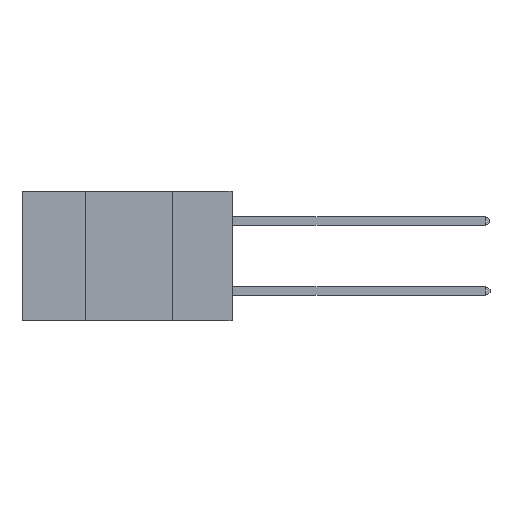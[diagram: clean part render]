
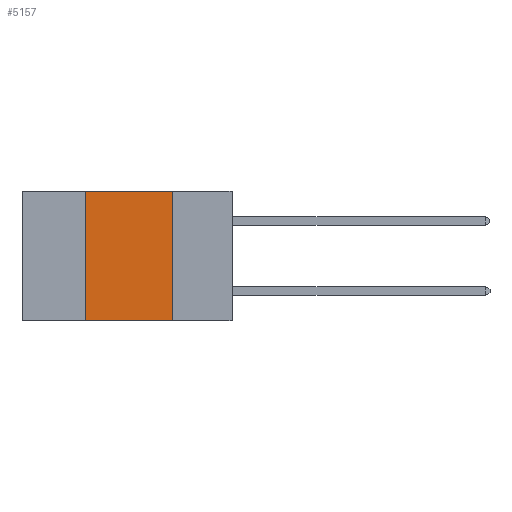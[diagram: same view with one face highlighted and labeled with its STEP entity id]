
A CAD part, left-side view. The second image highlights one B-rep face of the part: STEP entity #5157.
In plain terms, the highlighted planar face has unit normal (-1, 0, 0).
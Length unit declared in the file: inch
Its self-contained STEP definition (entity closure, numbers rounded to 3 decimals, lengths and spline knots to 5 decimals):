
#440 = CARTESIAN_POINT ( 'NONE',  ( 0., 0.17, 0. ) ) ;
#542 = LINE ( 'NONE', #7046, #11362 ) ;
#865 = VECTOR ( 'NONE', #4692, 39.37008 ) ;
#1323 = VECTOR ( 'NONE', #11215, 39.37008 ) ;
#1494 = CARTESIAN_POINT ( 'NONE',  ( 0., 0.42, 0. ) ) ;
#1680 = ORIENTED_EDGE ( 'NONE', *, *, #3179, .T. ) ;
#2598 = VERTEX_POINT ( 'NONE', #9716 ) ;
#2772 = LINE ( 'NONE', #6446, #13389 ) ;
#2850 = CARTESIAN_POINT ( 'NONE',  ( 0., 0.6, 0. ) ) ;
#3138 = EDGE_CURVE ( 'NONE', #6666, #8496, #542, .T. ) ;
#3179 = EDGE_CURVE ( 'NONE', #6666, #6652, #2772, .T. ) ;
#3407 = DIRECTION ( 'NONE',  ( 0., -1., 0. ) ) ;
#3831 = LINE ( 'NONE', #5006, #1323 ) ;
#3889 = DIRECTION ( 'NONE',  ( 0., 0., -1. ) ) ;
#3923 = EDGE_CURVE ( 'NONE', #2598, #6652, #4051, .T. ) ;
#4051 = LINE ( 'NONE', #440, #865 ) ;
#4070 = EDGE_CURVE ( 'NONE', #8496, #2598, #3831, .T. ) ;
#4692 = DIRECTION ( 'NONE',  ( 0., 0., -1. ) ) ;
#5006 = CARTESIAN_POINT ( 'NONE',  ( 0., 0.6, 0. ) ) ;
#5157 = ADVANCED_FACE ( 'NONE', ( #9524 ), #5947, .F. ) ;
#5915 = AXIS2_PLACEMENT_3D ( 'NONE', #2850, #10144, #3889 ) ;
#5947 = PLANE ( 'NONE',  #5915 ) ;
#6446 = CARTESIAN_POINT ( 'NONE',  ( 0., 0.6, -0.37 ) ) ;
#6652 = VERTEX_POINT ( 'NONE', #13172 ) ;
#6666 = VERTEX_POINT ( 'NONE', #9187 ) ;
#7046 = CARTESIAN_POINT ( 'NONE',  ( 0., 0.42, 0. ) ) ;
#7932 = ORIENTED_EDGE ( 'NONE', *, *, #4070, .F. ) ;
#8443 = DIRECTION ( 'NONE',  ( 0., 0., 1. ) ) ;
#8496 = VERTEX_POINT ( 'NONE', #1494 ) ;
#9168 = EDGE_LOOP ( 'NONE', ( #10353, #7932, #12245, #1680 ) ) ;
#9187 = CARTESIAN_POINT ( 'NONE',  ( 0., 0.42, -0.37 ) ) ;
#9524 = FACE_OUTER_BOUND ( 'NONE', #9168, .T. ) ;
#9716 = CARTESIAN_POINT ( 'NONE',  ( 0., 0.17, 0. ) ) ;
#10144 = DIRECTION ( 'NONE',  ( 1., 0., 0. ) ) ;
#10353 = ORIENTED_EDGE ( 'NONE', *, *, #3923, .F. ) ;
#11215 = DIRECTION ( 'NONE',  ( 0., -1., 0. ) ) ;
#11362 = VECTOR ( 'NONE', #8443, 39.37008 ) ;
#12245 = ORIENTED_EDGE ( 'NONE', *, *, #3138, .F. ) ;
#13172 = CARTESIAN_POINT ( 'NONE',  ( 0., 0.17, -0.37 ) ) ;
#13389 = VECTOR ( 'NONE', #3407, 39.37008 ) ;
